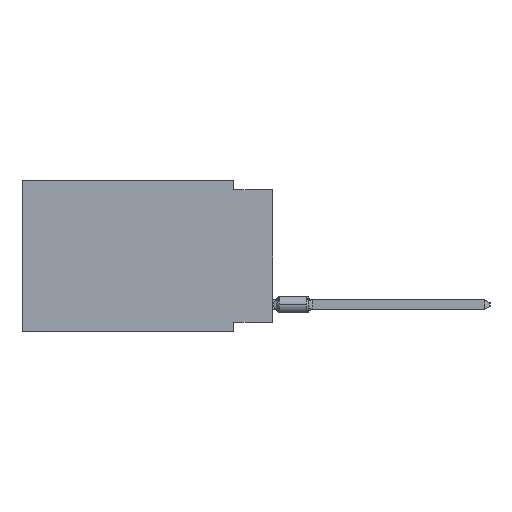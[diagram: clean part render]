
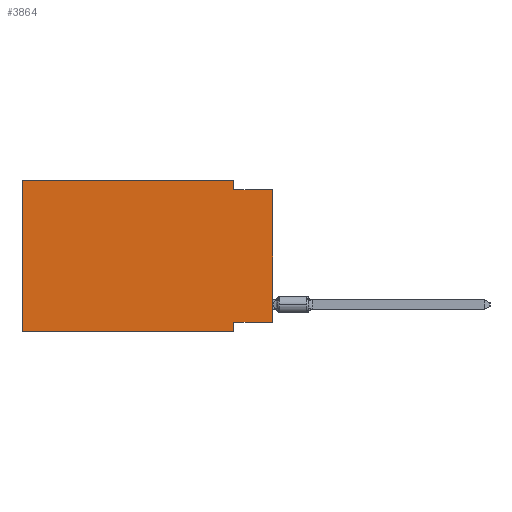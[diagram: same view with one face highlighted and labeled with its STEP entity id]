
A CAD part, left-side view. The second image highlights one B-rep face of the part: STEP entity #3864.
In plain terms, the highlighted planar face has unit normal (-1, 0, 0).
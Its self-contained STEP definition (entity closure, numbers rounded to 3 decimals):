
#1409 = CARTESIAN_POINT ( 'NONE',  ( 0., 16.383, 0. ) ) ;
#1680 = CARTESIAN_POINT ( 'NONE',  ( 0., 16.383, 0. ) ) ;
#1780 = CARTESIAN_POINT ( 'NONE',  ( 0., 16.383, -9.906 ) ) ;
#1838 = VECTOR ( 'NONE', #2787, 1000. ) ;
#2538 = CARTESIAN_POINT ( 'NONE',  ( 0., 2.54, 0. ) ) ;
#2787 = DIRECTION ( 'NONE',  ( 0., -1., 0. ) ) ;
#3005 = EDGE_LOOP ( 'NONE', ( #10279, #28075, #10286, #18724, #22764, #24527, #4986, #10709 ) ) ;
#3141 = LINE ( 'NONE', #17676, #19484 ) ;
#3740 = LINE ( 'NONE', #1409, #14726 ) ;
#3864 = ADVANCED_FACE ( 'NONE', ( #10393 ), #5123, .F. ) ;
#4986 = ORIENTED_EDGE ( 'NONE', *, *, #13375, .F. ) ;
#5123 = PLANE ( 'NONE',  #15617 ) ;
#5356 = VECTOR ( 'NONE', #17014, 1000. ) ;
#6115 = CARTESIAN_POINT ( 'NONE',  ( 0., 0., -9.271 ) ) ;
#6654 = CARTESIAN_POINT ( 'NONE',  ( 0., 0., -0.635 ) ) ;
#6716 = EDGE_CURVE ( 'NONE', #24634, #25567, #23098, .T. ) ;
#6884 = LINE ( 'NONE', #2538, #27310 ) ;
#7163 = VERTEX_POINT ( 'NONE', #18399 ) ;
#7516 = EDGE_CURVE ( 'NONE', #24634, #26535, #23301, .T. ) ;
#9198 = EDGE_CURVE ( 'NONE', #21525, #29741, #19343, .T. ) ;
#9330 = EDGE_CURVE ( 'NONE', #24521, #29741, #28642, .T. ) ;
#9632 = CARTESIAN_POINT ( 'NONE',  ( 0., 2.54, -9.906 ) ) ;
#10279 = ORIENTED_EDGE ( 'NONE', *, *, #9198, .T. ) ;
#10286 = ORIENTED_EDGE ( 'NONE', *, *, #29037, .F. ) ;
#10393 = FACE_OUTER_BOUND ( 'NONE', #3005, .T. ) ;
#10709 = ORIENTED_EDGE ( 'NONE', *, *, #28447, .F. ) ;
#10883 = CARTESIAN_POINT ( 'NONE',  ( 0., 16.383, -9.906 ) ) ;
#11364 = VERTEX_POINT ( 'NONE', #12581 ) ;
#12580 = DIRECTION ( 'NONE',  ( 0., 0., -1. ) ) ;
#12581 = CARTESIAN_POINT ( 'NONE',  ( 0., 2.54, 0. ) ) ;
#13375 = EDGE_CURVE ( 'NONE', #7163, #26535, #3141, .T. ) ;
#14515 = DIRECTION ( 'NONE',  ( 0., 1., 0. ) ) ;
#14726 = VECTOR ( 'NONE', #29275, 1000. ) ;
#14863 = CARTESIAN_POINT ( 'NONE',  ( 0., 0., 0. ) ) ;
#15617 = AXIS2_PLACEMENT_3D ( 'NONE', #21990, #19509, #26640 ) ;
#16325 = DIRECTION ( 'NONE',  ( 0., 0., -1. ) ) ;
#16890 = VECTOR ( 'NONE', #27434, 1000. ) ;
#17014 = DIRECTION ( 'NONE',  ( 0., 0., 1. ) ) ;
#17330 = CARTESIAN_POINT ( 'NONE',  ( 0., 0., -0.635 ) ) ;
#17676 = CARTESIAN_POINT ( 'NONE',  ( 0., 2.54, -9.906 ) ) ;
#18399 = CARTESIAN_POINT ( 'NONE',  ( 0., 2.54, -9.271 ) ) ;
#18724 = ORIENTED_EDGE ( 'NONE', *, *, #20207, .F. ) ;
#19343 = LINE ( 'NONE', #14863, #5356 ) ;
#19484 = VECTOR ( 'NONE', #12580, 1000. ) ;
#19509 = DIRECTION ( 'NONE',  ( 1., 0., 0. ) ) ;
#20207 = EDGE_CURVE ( 'NONE', #25567, #11364, #3740, .T. ) ;
#21264 = DIRECTION ( 'NONE',  ( 0., -1., 0. ) ) ;
#21525 = VERTEX_POINT ( 'NONE', #6115 ) ;
#21941 = CARTESIAN_POINT ( 'NONE',  ( 0., 0., -9.271 ) ) ;
#21990 = CARTESIAN_POINT ( 'NONE',  ( 0., 16.383, 0. ) ) ;
#22764 = ORIENTED_EDGE ( 'NONE', *, *, #6716, .F. ) ;
#22790 = CARTESIAN_POINT ( 'NONE',  ( 0., 2.54, -0.635 ) ) ;
#23098 = LINE ( 'NONE', #25115, #16890 ) ;
#23301 = LINE ( 'NONE', #1780, #25076 ) ;
#24521 = VERTEX_POINT ( 'NONE', #22790 ) ;
#24527 = ORIENTED_EDGE ( 'NONE', *, *, #7516, .T. ) ;
#24634 = VERTEX_POINT ( 'NONE', #10883 ) ;
#24811 = VECTOR ( 'NONE', #14515, 1000. ) ;
#25076 = VECTOR ( 'NONE', #21264, 1000. ) ;
#25115 = CARTESIAN_POINT ( 'NONE',  ( 0., 16.383, 0. ) ) ;
#25567 = VERTEX_POINT ( 'NONE', #1680 ) ;
#26535 = VERTEX_POINT ( 'NONE', #9632 ) ;
#26640 = DIRECTION ( 'NONE',  ( 0., 0., -1. ) ) ;
#27310 = VECTOR ( 'NONE', #16325, 1000. ) ;
#27434 = DIRECTION ( 'NONE',  ( 0., 0., 1. ) ) ;
#28075 = ORIENTED_EDGE ( 'NONE', *, *, #9330, .F. ) ;
#28447 = EDGE_CURVE ( 'NONE', #21525, #7163, #28912, .T. ) ;
#28642 = LINE ( 'NONE', #17330, #1838 ) ;
#28912 = LINE ( 'NONE', #21941, #24811 ) ;
#29037 = EDGE_CURVE ( 'NONE', #11364, #24521, #6884, .T. ) ;
#29275 = DIRECTION ( 'NONE',  ( 0., -1., 0. ) ) ;
#29741 = VERTEX_POINT ( 'NONE', #6654 ) ;
